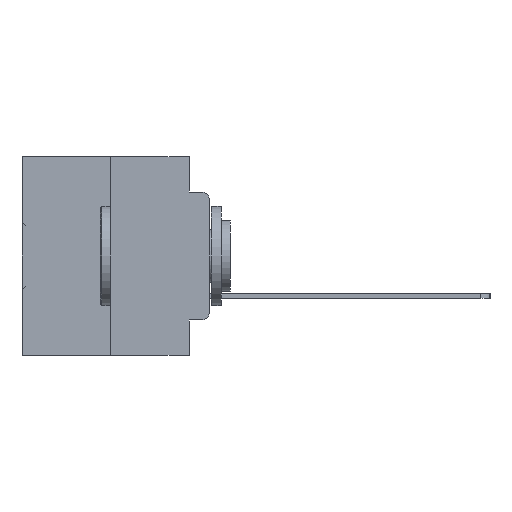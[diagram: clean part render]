
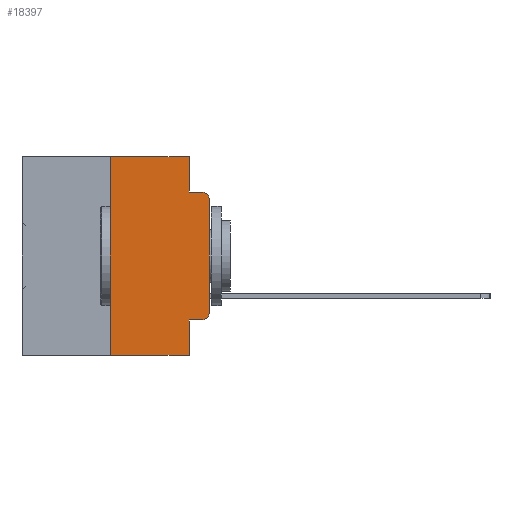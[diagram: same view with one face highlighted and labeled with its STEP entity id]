
A CAD part, left-side view. The second image highlights one B-rep face of the part: STEP entity #18397.
In plain terms, the highlighted planar face has unit normal (-1, 0, 0).
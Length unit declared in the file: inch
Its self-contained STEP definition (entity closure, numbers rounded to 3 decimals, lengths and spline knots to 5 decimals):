
#18 = PLANE ( 'NONE',  #32024 ) ;
#201 = CARTESIAN_POINT ( 'NONE',  ( 0., 0.051, -0.4115 ) ) ;
#1806 = ORIENTED_EDGE ( 'NONE', *, *, #11040, .F. ) ;
#1949 = CARTESIAN_POINT ( 'NONE',  ( 0., 0.051, -0.5 ) ) ;
#2645 = ORIENTED_EDGE ( 'NONE', *, *, #14883, .T. ) ;
#3080 = DIRECTION ( 'NONE',  ( 0., 0., 1. ) ) ;
#3492 = VERTEX_POINT ( 'NONE', #14097 ) ;
#3531 = DIRECTION ( 'NONE',  ( 0., 0., 1. ) ) ;
#4000 = ORIENTED_EDGE ( 'NONE', *, *, #5555, .F. ) ;
#4316 = CIRCLE ( 'NONE', #9013, 0.02 ) ;
#4361 = ORIENTED_EDGE ( 'NONE', *, *, #21083, .F. ) ;
#4996 = EDGE_LOOP ( 'NONE', ( #14959, #12869, #4361, #30274, #13339, #4000, #24618, #1806, #2645, #14528 ) ) ;
#5555 = EDGE_CURVE ( 'NONE', #22178, #21669, #16281, .T. ) ;
#5605 = DIRECTION ( 'NONE',  ( 0., 0., -1. ) ) ;
#5743 = VECTOR ( 'NONE', #27007, 39.37008 ) ;
#5885 = VECTOR ( 'NONE', #3531, 39.37008 ) ;
#6545 = VERTEX_POINT ( 'NONE', #7849 ) ;
#6606 = VECTOR ( 'NONE', #22151, 39.37008 ) ;
#7592 = VERTEX_POINT ( 'NONE', #26863 ) ;
#7704 = CARTESIAN_POINT ( 'NONE',  ( 0., 0.473, -0.5 ) ) ;
#7762 = VECTOR ( 'NONE', #33657, 39.37008 ) ;
#7849 = CARTESIAN_POINT ( 'NONE',  ( 0., 0.051, 0. ) ) ;
#9013 = AXIS2_PLACEMENT_3D ( 'NONE', #31644, #15768, #34290 ) ;
#9068 = VECTOR ( 'NONE', #3080, 39.37008 ) ;
#9872 = EDGE_CURVE ( 'NONE', #31807, #24042, #10544, .T. ) ;
#10544 = CIRCLE ( 'NONE', #14393, 0.02 ) ;
#10863 = VERTEX_POINT ( 'NONE', #1949 ) ;
#11040 = EDGE_CURVE ( 'NONE', #30499, #10863, #19262, .T. ) ;
#11230 = CARTESIAN_POINT ( 'NONE',  ( 0., 0.25, 0. ) ) ;
#11556 = EDGE_CURVE ( 'NONE', #22178, #10863, #13218, .T. ) ;
#11699 = CARTESIAN_POINT ( 'NONE',  ( 0., 0.02, -0.0885 ) ) ;
#12869 = ORIENTED_EDGE ( 'NONE', *, *, #9872, .T. ) ;
#13018 = LINE ( 'NONE', #18997, #5743 ) ;
#13178 = DIRECTION ( 'NONE',  ( 0., -1., 0. ) ) ;
#13194 = VECTOR ( 'NONE', #16028, 39.37008 ) ;
#13208 = EDGE_CURVE ( 'NONE', #27051, #31807, #17765, .T. ) ;
#13218 = LINE ( 'NONE', #7704, #19476 ) ;
#13298 = LINE ( 'NONE', #15120, #7762 ) ;
#13334 = CARTESIAN_POINT ( 'NONE',  ( 0., 0.051, -0.0885 ) ) ;
#13339 = ORIENTED_EDGE ( 'NONE', *, *, #16745, .F. ) ;
#14097 = CARTESIAN_POINT ( 'NONE',  ( 0., 0.051, -0.0885 ) ) ;
#14393 = AXIS2_PLACEMENT_3D ( 'NONE', #31057, #15180, #33720 ) ;
#14528 = ORIENTED_EDGE ( 'NONE', *, *, #19785, .T. ) ;
#14883 = EDGE_CURVE ( 'NONE', #30499, #7592, #13018, .T. ) ;
#14959 = ORIENTED_EDGE ( 'NONE', *, *, #13208, .T. ) ;
#15120 = CARTESIAN_POINT ( 'NONE',  ( 0., 0.473, 0. ) ) ;
#15180 = DIRECTION ( 'NONE',  ( -1., 0., 0. ) ) ;
#15527 = VECTOR ( 'NONE', #18958, 39.37008 ) ;
#15768 = DIRECTION ( 'NONE',  ( -1., 0., 0. ) ) ;
#16028 = DIRECTION ( 'NONE',  ( 0., -1., 0. ) ) ;
#16281 = LINE ( 'NONE', #11230, #9068 ) ;
#16745 = EDGE_CURVE ( 'NONE', #21669, #6545, #13298, .T. ) ;
#16801 = CARTESIAN_POINT ( 'NONE',  ( 0., 0.051, 0. ) ) ;
#17765 = LINE ( 'NONE', #19776, #5885 ) ;
#18397 = ADVANCED_FACE ( 'NONE', ( #21681 ), #18, .F. ) ;
#18958 = DIRECTION ( 'NONE',  ( 0., 0., -1. ) ) ;
#18997 = CARTESIAN_POINT ( 'NONE',  ( 0., 0.051, -0.4115 ) ) ;
#19105 = CARTESIAN_POINT ( 'NONE',  ( 0., 0.473, 0. ) ) ;
#19262 = LINE ( 'NONE', #34760, #15527 ) ;
#19476 = VECTOR ( 'NONE', #13178, 39.37008 ) ;
#19776 = CARTESIAN_POINT ( 'NONE',  ( 0., 0., 0. ) ) ;
#19785 = EDGE_CURVE ( 'NONE', #7592, #27051, #4316, .T. ) ;
#21083 = EDGE_CURVE ( 'NONE', #3492, #24042, #34350, .T. ) ;
#21669 = VERTEX_POINT ( 'NONE', #25192 ) ;
#21681 = FACE_OUTER_BOUND ( 'NONE', #4996, .T. ) ;
#21758 = DIRECTION ( 'NONE',  ( 1., 0., 0. ) ) ;
#22151 = DIRECTION ( 'NONE',  ( 0., 0., -1. ) ) ;
#22178 = VERTEX_POINT ( 'NONE', #24690 ) ;
#23487 = EDGE_CURVE ( 'NONE', #6545, #3492, #33388, .T. ) ;
#24042 = VERTEX_POINT ( 'NONE', #11699 ) ;
#24618 = ORIENTED_EDGE ( 'NONE', *, *, #11556, .T. ) ;
#24690 = CARTESIAN_POINT ( 'NONE',  ( 0., 0.25, -0.5 ) ) ;
#25192 = CARTESIAN_POINT ( 'NONE',  ( 0., 0.25, 0. ) ) ;
#26863 = CARTESIAN_POINT ( 'NONE',  ( 0., 0.02, -0.4115 ) ) ;
#27007 = DIRECTION ( 'NONE',  ( 0., -1., 0. ) ) ;
#27051 = VERTEX_POINT ( 'NONE', #30027 ) ;
#30027 = CARTESIAN_POINT ( 'NONE',  ( 0., 0., -0.3915 ) ) ;
#30161 = CARTESIAN_POINT ( 'NONE',  ( 0., 0., -0.1085 ) ) ;
#30274 = ORIENTED_EDGE ( 'NONE', *, *, #23487, .F. ) ;
#30499 = VERTEX_POINT ( 'NONE', #201 ) ;
#31057 = CARTESIAN_POINT ( 'NONE',  ( 0., 0.02, -0.1085 ) ) ;
#31644 = CARTESIAN_POINT ( 'NONE',  ( 0., 0.02, -0.3915 ) ) ;
#31807 = VERTEX_POINT ( 'NONE', #30161 ) ;
#32024 = AXIS2_PLACEMENT_3D ( 'NONE', #19105, #21758, #5605 ) ;
#33388 = LINE ( 'NONE', #16801, #6606 ) ;
#33657 = DIRECTION ( 'NONE',  ( 0., -1., 0. ) ) ;
#33720 = DIRECTION ( 'NONE',  ( 0., 0., -1. ) ) ;
#34290 = DIRECTION ( 'NONE',  ( 0., 0., -1. ) ) ;
#34350 = LINE ( 'NONE', #13334, #13194 ) ;
#34760 = CARTESIAN_POINT ( 'NONE',  ( 0., 0.051, 0. ) ) ;
